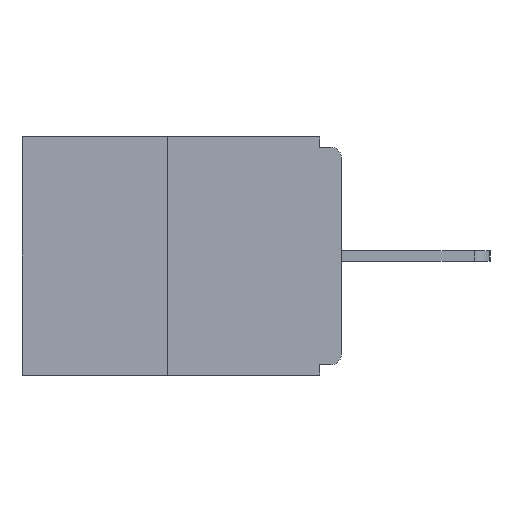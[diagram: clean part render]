
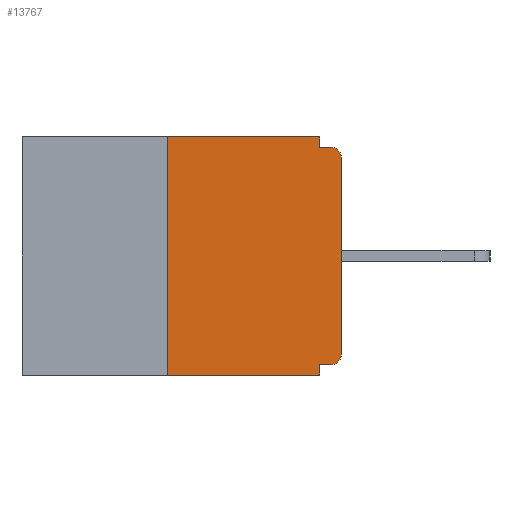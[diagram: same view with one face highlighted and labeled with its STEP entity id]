
A CAD part, left-side view. The second image highlights one B-rep face of the part: STEP entity #13767.
In plain terms, the highlighted planar face has unit normal (-1, 0, 0).
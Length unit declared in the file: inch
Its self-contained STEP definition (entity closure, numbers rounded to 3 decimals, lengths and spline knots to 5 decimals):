
#22 = VECTOR ( 'NONE', #9494, 39.37008 ) ;
#95 = ORIENTED_EDGE ( 'NONE', *, *, #8345, .F. ) ;
#396 = CARTESIAN_POINT ( 'NONE',  ( 0., 0.015, -0.313 ) ) ;
#437 = AXIS2_PLACEMENT_3D ( 'NONE', #6522, #7565, #11851 ) ;
#513 = EDGE_CURVE ( 'NONE', #1785, #9585, #6271, .T. ) ;
#600 = PLANE ( 'NONE',  #753 ) ;
#719 = EDGE_CURVE ( 'NONE', #9735, #9308, #12072, .T. ) ;
#726 = VECTOR ( 'NONE', #5727, 39.37008 ) ;
#753 = AXIS2_PLACEMENT_3D ( 'NONE', #4848, #4705, #7031 ) ;
#1085 = CARTESIAN_POINT ( 'NONE',  ( 0., 0.031, -0.328 ) ) ;
#1149 = VECTOR ( 'NONE', #3604, 39.37008 ) ;
#1323 = CARTESIAN_POINT ( 'NONE',  ( 0., 0., -0.313 ) ) ;
#1785 = VERTEX_POINT ( 'NONE', #7006 ) ;
#1965 = CARTESIAN_POINT ( 'NONE',  ( 0., 0., -0.03 ) ) ;
#2020 = LINE ( 'NONE', #9356, #22 ) ;
#2256 = EDGE_CURVE ( 'NONE', #3614, #9585, #5785, .T. ) ;
#2446 = DIRECTION ( 'NONE',  ( 0., 0., -1. ) ) ;
#2503 = VECTOR ( 'NONE', #9518, 39.37008 ) ;
#2628 = ORIENTED_EDGE ( 'NONE', *, *, #2256, .T. ) ;
#2788 = CARTESIAN_POINT ( 'NONE',  ( 0., 0.015, -0.015 ) ) ;
#2882 = DIRECTION ( 'NONE',  ( 0., -1., 0. ) ) ;
#3133 = CARTESIAN_POINT ( 'NONE',  ( 0., 0.031, 0. ) ) ;
#3152 = EDGE_CURVE ( 'NONE', #13339, #3614, #4187, .T. ) ;
#3604 = DIRECTION ( 'NONE',  ( 0., -1., 0. ) ) ;
#3614 = VERTEX_POINT ( 'NONE', #1965 ) ;
#3633 = DIRECTION ( 'NONE',  ( -1., 0., 0. ) ) ;
#3745 = CARTESIAN_POINT ( 'NONE',  ( 0., 0.46, 0. ) ) ;
#3975 = EDGE_CURVE ( 'NONE', #8003, #9735, #2020, .T. ) ;
#4187 = LINE ( 'NONE', #9571, #2503 ) ;
#4588 = CARTESIAN_POINT ( 'NONE',  ( 0., 0.25, -0.343 ) ) ;
#4705 = DIRECTION ( 'NONE',  ( 1., 0., 0. ) ) ;
#4848 = CARTESIAN_POINT ( 'NONE',  ( 0., 0.46, 0. ) ) ;
#4979 = ORIENTED_EDGE ( 'NONE', *, *, #10815, .T. ) ;
#4986 = EDGE_CURVE ( 'NONE', #8003, #13339, #5178, .T. ) ;
#5178 = CIRCLE ( 'NONE', #6255, 0.015 ) ;
#5304 = VECTOR ( 'NONE', #2882, 39.37008 ) ;
#5727 = DIRECTION ( 'NONE',  ( 0., 0., 1. ) ) ;
#5747 = DIRECTION ( 'NONE',  ( 0., -1., 0. ) ) ;
#5785 = CIRCLE ( 'NONE', #437, 0.015 ) ;
#6255 = AXIS2_PLACEMENT_3D ( 'NONE', #396, #3633, #2446 ) ;
#6271 = LINE ( 'NONE', #11392, #5304 ) ;
#6518 = EDGE_CURVE ( 'NONE', #13394, #1785, #11804, .T. ) ;
#6522 = CARTESIAN_POINT ( 'NONE',  ( 0., 0.015, -0.03 ) ) ;
#6597 = CARTESIAN_POINT ( 'NONE',  ( 0., 0.46, -0.343 ) ) ;
#6614 = VERTEX_POINT ( 'NONE', #12218 ) ;
#6958 = VECTOR ( 'NONE', #10755, 39.37008 ) ;
#6962 = DIRECTION ( 'NONE',  ( 0., 0., -1. ) ) ;
#7006 = CARTESIAN_POINT ( 'NONE',  ( 0., 0.031, -0.015 ) ) ;
#7031 = DIRECTION ( 'NONE',  ( 0., 0., -1. ) ) ;
#7383 = CARTESIAN_POINT ( 'NONE',  ( 0., 0.031, -0.343 ) ) ;
#7565 = DIRECTION ( 'NONE',  ( -1., 0., 0. ) ) ;
#7857 = LINE ( 'NONE', #6597, #1149 ) ;
#7922 = ORIENTED_EDGE ( 'NONE', *, *, #3975, .F. ) ;
#7924 = FACE_OUTER_BOUND ( 'NONE', #12271, .T. ) ;
#8003 = VERTEX_POINT ( 'NONE', #8225 ) ;
#8225 = CARTESIAN_POINT ( 'NONE',  ( 0., 0.015, -0.328 ) ) ;
#8345 = EDGE_CURVE ( 'NONE', #6614, #13394, #9202, .T. ) ;
#8775 = CARTESIAN_POINT ( 'NONE',  ( 0., 0.031, -0.343 ) ) ;
#9046 = VERTEX_POINT ( 'NONE', #4588 ) ;
#9202 = LINE ( 'NONE', #3745, #10350 ) ;
#9308 = VERTEX_POINT ( 'NONE', #7383 ) ;
#9315 = ORIENTED_EDGE ( 'NONE', *, *, #719, .F. ) ;
#9356 = CARTESIAN_POINT ( 'NONE',  ( 0., 0., -0.328 ) ) ;
#9494 = DIRECTION ( 'NONE',  ( 0., 1., 0. ) ) ;
#9518 = DIRECTION ( 'NONE',  ( 0., 0., 1. ) ) ;
#9571 = CARTESIAN_POINT ( 'NONE',  ( 0., 0., 0. ) ) ;
#9585 = VERTEX_POINT ( 'NONE', #2788 ) ;
#9735 = VERTEX_POINT ( 'NONE', #1085 ) ;
#9937 = ORIENTED_EDGE ( 'NONE', *, *, #12795, .F. ) ;
#10350 = VECTOR ( 'NONE', #5747, 39.37008 ) ;
#10718 = ORIENTED_EDGE ( 'NONE', *, *, #6518, .F. ) ;
#10755 = DIRECTION ( 'NONE',  ( 0., 0., -1. ) ) ;
#10815 = EDGE_CURVE ( 'NONE', #9046, #9308, #7857, .T. ) ;
#10849 = ORIENTED_EDGE ( 'NONE', *, *, #3152, .T. ) ;
#10917 = CARTESIAN_POINT ( 'NONE',  ( 0., 0.25, 0. ) ) ;
#11172 = ORIENTED_EDGE ( 'NONE', *, *, #4986, .T. ) ;
#11392 = CARTESIAN_POINT ( 'NONE',  ( 0., 0., -0.015 ) ) ;
#11616 = VECTOR ( 'NONE', #6962, 39.37008 ) ;
#11804 = LINE ( 'NONE', #3133, #6958 ) ;
#11851 = DIRECTION ( 'NONE',  ( 0., 0., -1. ) ) ;
#12072 = LINE ( 'NONE', #8775, #11616 ) ;
#12125 = LINE ( 'NONE', #10917, #726 ) ;
#12218 = CARTESIAN_POINT ( 'NONE',  ( 0., 0.25, 0. ) ) ;
#12271 = EDGE_LOOP ( 'NONE', ( #95, #9937, #4979, #9315, #7922, #11172, #10849, #2628, #13114, #10718 ) ) ;
#12523 = CARTESIAN_POINT ( 'NONE',  ( 0., 0.031, 0. ) ) ;
#12795 = EDGE_CURVE ( 'NONE', #9046, #6614, #12125, .T. ) ;
#13114 = ORIENTED_EDGE ( 'NONE', *, *, #513, .F. ) ;
#13339 = VERTEX_POINT ( 'NONE', #1323 ) ;
#13394 = VERTEX_POINT ( 'NONE', #12523 ) ;
#13767 = ADVANCED_FACE ( 'NONE', ( #7924 ), #600, .F. ) ;
